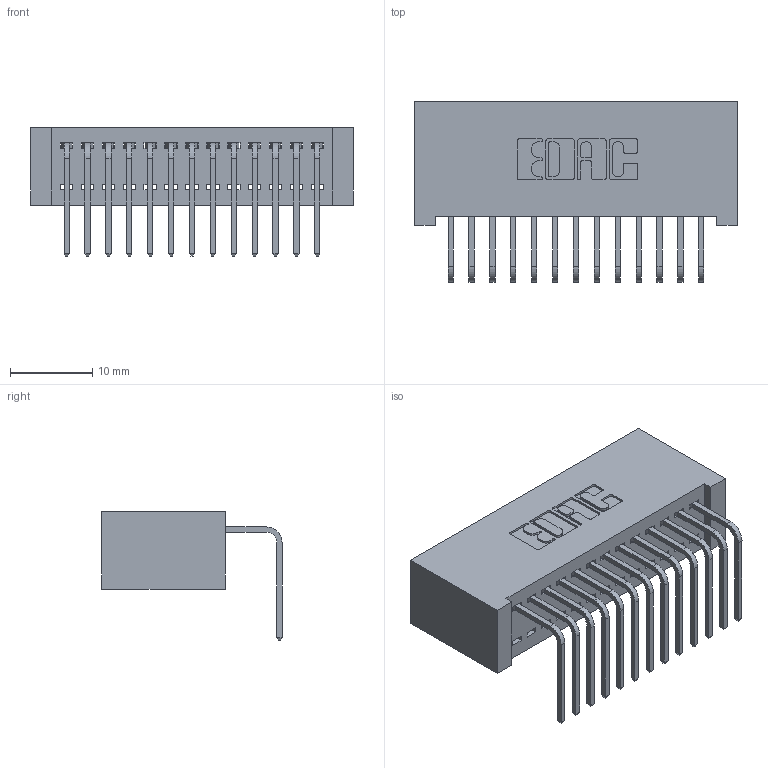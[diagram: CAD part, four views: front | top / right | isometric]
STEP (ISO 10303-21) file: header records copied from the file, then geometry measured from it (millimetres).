
FILE_DESCRIPTION (( 'STEP AP203' ), '1' );
FILE_NAME ('392-013-558-101.STEP', '2019-10-07T01:59:01', ( '' ), ( '' ), 'SwSTEP 2.0', 'SolidWorks 2016', '' );
FILE_SCHEMA (( 'CONFIG_CONTROL_DESIGN' ));
Length unit declared in the file: inch
Products named in the file (3): 392-013-558-101; 342 Part_Lugless; 345-292-001_558 Tail - 2
Assembly tree (14 placements, depth 2):
  392-013-558-101
    342 Part_Lugless
    345-292-001_558 Tail - 2  x13
Bounding box: 39.27 x 21.91 x 15.62 mm (x, y, z)
Volume: 3788.5 mm3; surface area: 5591.1 mm2
Topology: 14 solids, 14 shells, 882 faces, 2641 edges, 1742 vertices
Faces by surface type: plane 634, cylinder 248
Entity records: 11373 total; most frequent: CARTESIAN_POINT 1973, ORIENTED_EDGE 1922, DIRECTION 1715, EDGE_CURVE 961, LINE 841, VECTOR 841, VERTEX_POINT 638, AXIS2_PLACEMENT_3D 437
